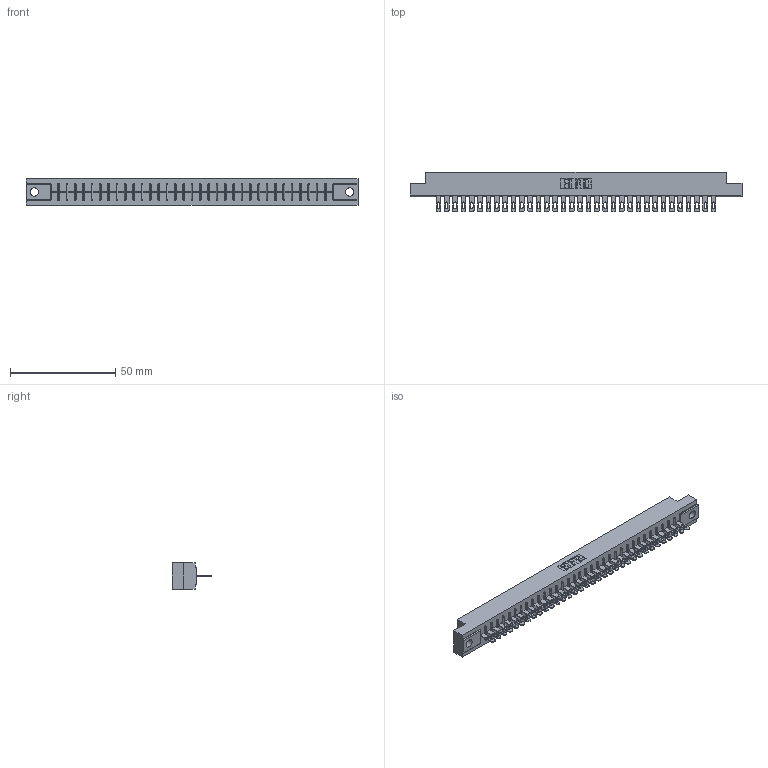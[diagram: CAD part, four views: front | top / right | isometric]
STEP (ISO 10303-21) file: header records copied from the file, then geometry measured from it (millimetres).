
FILE_DESCRIPTION (( 'STEP AP203' ), '1' );
FILE_NAME ('316-034-500-104.STEP', '2018-07-31T04:00:16', ( '' ), ( '' ), 'SwSTEP 2.0', 'SolidWorks 2016', '' );
FILE_SCHEMA (( 'CONFIG_CONTROL_DESIGN' ));
Length unit declared in the file: inch
Products named in the file (3): 306 Part_.156 Dia; 306-290-001_100; 316-034-500-104
Assembly tree (35 placements, depth 2):
  316-034-500-104
    306 Part_.156 Dia
    306-290-001_100  x34
Bounding box: 157.73 x 18.87 x 12.7 mm (x, y, z)
Volume: 17380.2 mm3; surface area: 18156.6 mm2
Topology: 35 solids, 35 shells, 2714 faces, 7662 edges, 4924 vertices
Faces by surface type: plane 1782, cylinder 796, sphere 136
Entity records: 33325 total; most frequent: CARTESIAN_POINT 5599, ORIENTED_EDGE 5548, DIRECTION 5514, EDGE_CURVE 2774, VECTOR 2172, LINE 2172, VERTEX_POINT 1756, AXIS2_PLACEMENT_3D 1671
